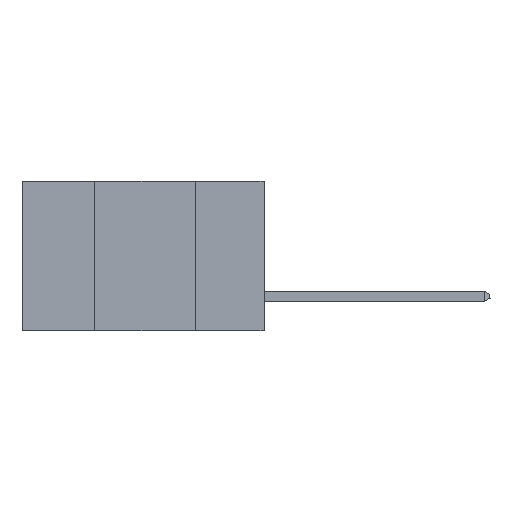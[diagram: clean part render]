
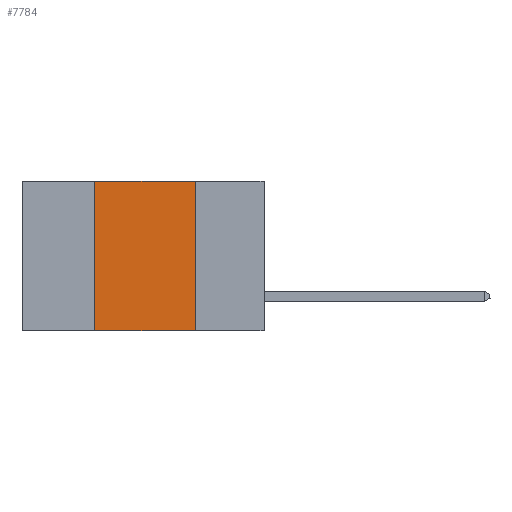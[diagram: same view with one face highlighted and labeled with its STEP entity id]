
A CAD part, left-side view. The second image highlights one B-rep face of the part: STEP entity #7784.
In plain terms, the highlighted planar face has unit normal (-1, 0, 0).
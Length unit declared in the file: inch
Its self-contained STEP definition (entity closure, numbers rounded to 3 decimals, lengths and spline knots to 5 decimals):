
#1368 = VECTOR ( 'NONE', #23207, 39.37008 ) ;
#1390 = DIRECTION ( 'NONE',  ( 0., 0., 1. ) ) ;
#1499 = VECTOR ( 'NONE', #1390, 39.37008 ) ;
#1745 = VERTEX_POINT ( 'NONE', #10745 ) ;
#4205 = ORIENTED_EDGE ( 'NONE', *, *, #10384, .T. ) ;
#4206 = CARTESIAN_POINT ( 'NONE',  ( 0., 0.6, 0. ) ) ;
#4305 = DIRECTION ( 'NONE',  ( 0., -1., 0. ) ) ;
#4462 = LINE ( 'NONE', #22586, #19539 ) ;
#4715 = AXIS2_PLACEMENT_3D ( 'NONE', #21507, #23345, #10569 ) ;
#5969 = FACE_OUTER_BOUND ( 'NONE', #7091, .T. ) ;
#6416 = CARTESIAN_POINT ( 'NONE',  ( 0., 0.42, 0. ) ) ;
#6481 = ORIENTED_EDGE ( 'NONE', *, *, #23717, .F. ) ;
#6835 = EDGE_CURVE ( 'NONE', #25224, #12882, #12083, .T. ) ;
#7091 = EDGE_LOOP ( 'NONE', ( #12020, #6481, #20592, #4205 ) ) ;
#7434 = DIRECTION ( 'NONE',  ( 0., -1., 0. ) ) ;
#7784 = ADVANCED_FACE ( 'NONE', ( #5969 ), #14861, .F. ) ;
#10384 = EDGE_CURVE ( 'NONE', #1745, #12882, #4462, .T. ) ;
#10569 = DIRECTION ( 'NONE',  ( 0., 0., -1. ) ) ;
#10745 = CARTESIAN_POINT ( 'NONE',  ( 0., 0.42, -0.37 ) ) ;
#11722 = VECTOR ( 'NONE', #4305, 39.37008 ) ;
#12020 = ORIENTED_EDGE ( 'NONE', *, *, #6835, .F. ) ;
#12044 = LINE ( 'NONE', #4206, #11722 ) ;
#12083 = LINE ( 'NONE', #27214, #1368 ) ;
#12882 = VERTEX_POINT ( 'NONE', #14227 ) ;
#14227 = CARTESIAN_POINT ( 'NONE',  ( 0., 0.17, -0.37 ) ) ;
#14861 = PLANE ( 'NONE',  #4715 ) ;
#16415 = EDGE_CURVE ( 'NONE', #1745, #25107, #26257, .T. ) ;
#17662 = CARTESIAN_POINT ( 'NONE',  ( 0., 0.42, 0. ) ) ;
#19539 = VECTOR ( 'NONE', #7434, 39.37008 ) ;
#20592 = ORIENTED_EDGE ( 'NONE', *, *, #16415, .F. ) ;
#21507 = CARTESIAN_POINT ( 'NONE',  ( 0., 0.6, 0. ) ) ;
#22586 = CARTESIAN_POINT ( 'NONE',  ( 0., 0.6, -0.37 ) ) ;
#23207 = DIRECTION ( 'NONE',  ( 0., 0., -1. ) ) ;
#23345 = DIRECTION ( 'NONE',  ( 1., 0., 0. ) ) ;
#23717 = EDGE_CURVE ( 'NONE', #25107, #25224, #12044, .T. ) ;
#25107 = VERTEX_POINT ( 'NONE', #17662 ) ;
#25224 = VERTEX_POINT ( 'NONE', #26614 ) ;
#26257 = LINE ( 'NONE', #6416, #1499 ) ;
#26614 = CARTESIAN_POINT ( 'NONE',  ( 0., 0.17, 0. ) ) ;
#27214 = CARTESIAN_POINT ( 'NONE',  ( 0., 0.17, 0. ) ) ;
